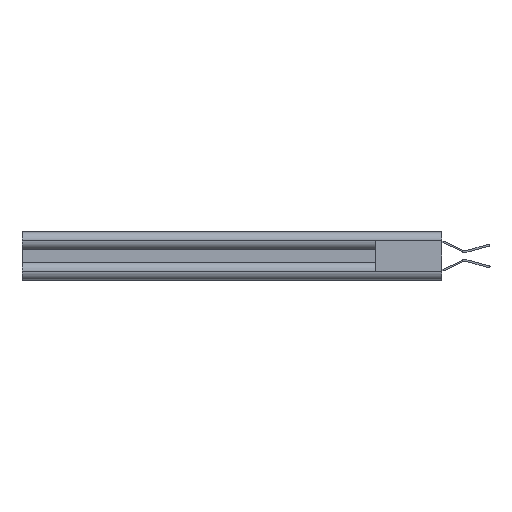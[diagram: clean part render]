
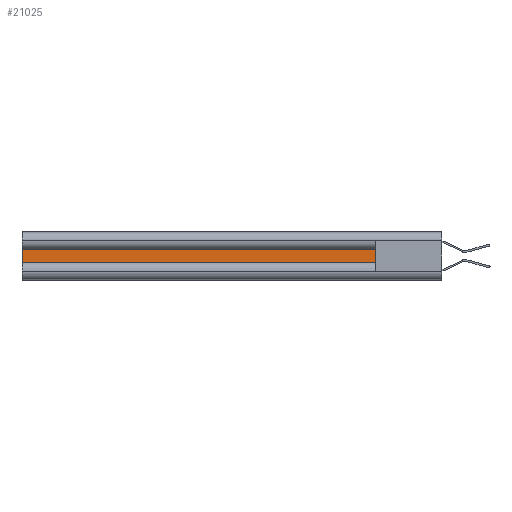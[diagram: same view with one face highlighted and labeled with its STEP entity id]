
A CAD part, left-side view. The second image highlights one B-rep face of the part: STEP entity #21025.
In plain terms, the highlighted planar face has unit normal (-1, 0, 0).
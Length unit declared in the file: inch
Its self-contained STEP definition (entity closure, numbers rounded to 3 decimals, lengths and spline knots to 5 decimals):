
#364 = LINE ( 'NONE', #2571, #8212 ) ;
#1405 = LINE ( 'NONE', #14122, #18690 ) ;
#1704 = ORIENTED_EDGE ( 'NONE', *, *, #10369, .F. ) ;
#1928 = VERTEX_POINT ( 'NONE', #13038 ) ;
#2571 = CARTESIAN_POINT ( 'NONE',  ( 0.044, 0.473, -0.0465 ) ) ;
#3213 = FACE_OUTER_BOUND ( 'NONE', #4228, .T. ) ;
#3541 = LINE ( 'NONE', #20924, #12183 ) ;
#3622 = CARTESIAN_POINT ( 'NONE',  ( 0.044, 0.473, -0.0465 ) ) ;
#4228 = EDGE_LOOP ( 'NONE', ( #14166, #9673, #1704, #10103 ) ) ;
#4371 = VERTEX_POINT ( 'NONE', #10674 ) ;
#5691 = PLANE ( 'NONE',  #16863 ) ;
#6145 = DIRECTION ( 'NONE',  ( 0., 0., -1. ) ) ;
#7047 = VERTEX_POINT ( 'NONE', #10871 ) ;
#7656 = EDGE_CURVE ( 'NONE', #4371, #1928, #3541, .T. ) ;
#8212 = VECTOR ( 'NONE', #6145, 39.37008 ) ;
#8430 = EDGE_CURVE ( 'NONE', #4371, #14572, #364, .T. ) ;
#8431 = LINE ( 'NONE', #21522, #21923 ) ;
#9673 = ORIENTED_EDGE ( 'NONE', *, *, #16247, .T. ) ;
#10103 = ORIENTED_EDGE ( 'NONE', *, *, #8430, .F. ) ;
#10369 = EDGE_CURVE ( 'NONE', #14572, #7047, #1405, .T. ) ;
#10674 = CARTESIAN_POINT ( 'NONE',  ( 0.044, 0.473, 0.0465 ) ) ;
#10841 = DIRECTION ( 'NONE',  ( 0., 0., -1. ) ) ;
#10871 = CARTESIAN_POINT ( 'NONE',  ( 0.044, 3., -0.0465 ) ) ;
#12183 = VECTOR ( 'NONE', #20996, 39.37008 ) ;
#13038 = CARTESIAN_POINT ( 'NONE',  ( 0.044, 3., 0.0465 ) ) ;
#14122 = CARTESIAN_POINT ( 'NONE',  ( 0.044, 0.37012, -0.0465 ) ) ;
#14166 = ORIENTED_EDGE ( 'NONE', *, *, #7656, .T. ) ;
#14572 = VERTEX_POINT ( 'NONE', #3622 ) ;
#14731 = DIRECTION ( 'NONE',  ( 0., 0., -1. ) ) ;
#15881 = DIRECTION ( 'NONE',  ( 0., 1., 0. ) ) ;
#16247 = EDGE_CURVE ( 'NONE', #1928, #7047, #8431, .T. ) ;
#16863 = AXIS2_PLACEMENT_3D ( 'NONE', #19198, #20984, #10841 ) ;
#18690 = VECTOR ( 'NONE', #15881, 39.37008 ) ;
#19198 = CARTESIAN_POINT ( 'NONE',  ( 0.044, 0.37012, -0.0465 ) ) ;
#20924 = CARTESIAN_POINT ( 'NONE',  ( 0.044, 0.37012, 0.0465 ) ) ;
#20984 = DIRECTION ( 'NONE',  ( 1., 0., 0. ) ) ;
#20996 = DIRECTION ( 'NONE',  ( 0., 1., 0. ) ) ;
#21025 = ADVANCED_FACE ( 'NONE', ( #3213 ), #5691, .F. ) ;
#21522 = CARTESIAN_POINT ( 'NONE',  ( 0.044, 3., -0.0465 ) ) ;
#21923 = VECTOR ( 'NONE', #14731, 39.37008 ) ;
